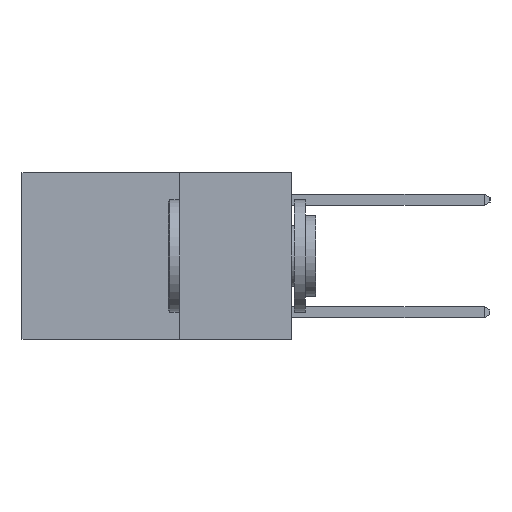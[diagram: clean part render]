
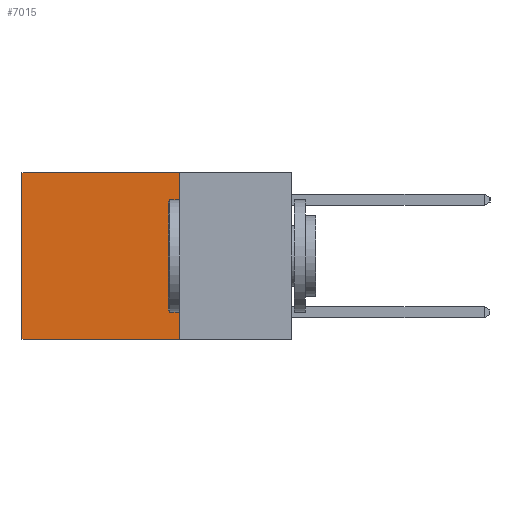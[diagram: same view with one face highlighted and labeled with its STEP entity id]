
A CAD part, left-side view. The second image highlights one B-rep face of the part: STEP entity #7015.
In plain terms, the highlighted planar face has unit normal (-1, 0, 0).
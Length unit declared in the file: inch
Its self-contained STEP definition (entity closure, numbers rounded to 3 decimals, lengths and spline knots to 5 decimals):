
#33 = ORIENTED_EDGE ( 'NONE', *, *, #1955, .F. ) ;
#361 = VERTEX_POINT ( 'NONE', #7771 ) ;
#423 = VERTEX_POINT ( 'NONE', #7670 ) ;
#875 = EDGE_LOOP ( 'NONE', ( #1395, #33, #5418, #2627 ) ) ;
#1241 = EDGE_CURVE ( 'NONE', #361, #423, #3917, .T. ) ;
#1385 = DIRECTION ( 'NONE',  ( 0., 0., -1. ) ) ;
#1395 = ORIENTED_EDGE ( 'NONE', *, *, #8363, .T. ) ;
#1513 = FACE_OUTER_BOUND ( 'NONE', #875, .T. ) ;
#1831 = CARTESIAN_POINT ( 'NONE',  ( 0.2625, 0.25, -0.37 ) ) ;
#1955 = EDGE_CURVE ( 'NONE', #423, #8313, #3493, .T. ) ;
#2224 = CARTESIAN_POINT ( 'NONE',  ( 0.2625, 0.25, 0. ) ) ;
#2562 = CARTESIAN_POINT ( 'NONE',  ( 0.2625, 0.6, -0.37 ) ) ;
#2627 = ORIENTED_EDGE ( 'NONE', *, *, #4364, .T. ) ;
#3493 = LINE ( 'NONE', #1831, #3540 ) ;
#3540 = VECTOR ( 'NONE', #7913, 39.37008 ) ;
#3891 = VECTOR ( 'NONE', #7590, 39.37008 ) ;
#3917 = LINE ( 'NONE', #5654, #3891 ) ;
#4248 = CARTESIAN_POINT ( 'NONE',  ( 0.2625, 0.25, 0. ) ) ;
#4364 = EDGE_CURVE ( 'NONE', #361, #4371, #7109, .T. ) ;
#4371 = VERTEX_POINT ( 'NONE', #6617 ) ;
#5418 = ORIENTED_EDGE ( 'NONE', *, *, #1241, .F. ) ;
#5654 = CARTESIAN_POINT ( 'NONE',  ( 0.2625, 0.25, 0. ) ) ;
#5785 = PLANE ( 'NONE',  #8905 ) ;
#6170 = LINE ( 'NONE', #8759, #6378 ) ;
#6378 = VECTOR ( 'NONE', #1385, 39.37008 ) ;
#6617 = CARTESIAN_POINT ( 'NONE',  ( 0.2625, 0.6, 0. ) ) ;
#6626 = DIRECTION ( 'NONE',  ( 0., 1., 0. ) ) ;
#6672 = DIRECTION ( 'NONE',  ( 1., 0., 0. ) ) ;
#7006 = VECTOR ( 'NONE', #6626, 39.37008 ) ;
#7015 = ADVANCED_FACE ( 'NONE', ( #1513 ), #5785, .F. ) ;
#7031 = DIRECTION ( 'NONE',  ( 0., 0., -1. ) ) ;
#7109 = LINE ( 'NONE', #4248, #7006 ) ;
#7590 = DIRECTION ( 'NONE',  ( 0., 0., -1. ) ) ;
#7670 = CARTESIAN_POINT ( 'NONE',  ( 0.2625, 0.25, -0.37 ) ) ;
#7771 = CARTESIAN_POINT ( 'NONE',  ( 0.2625, 0.25, 0. ) ) ;
#7913 = DIRECTION ( 'NONE',  ( 0., 1., 0. ) ) ;
#8313 = VERTEX_POINT ( 'NONE', #2562 ) ;
#8363 = EDGE_CURVE ( 'NONE', #4371, #8313, #6170, .T. ) ;
#8759 = CARTESIAN_POINT ( 'NONE',  ( 0.2625, 0.6, 0. ) ) ;
#8905 = AXIS2_PLACEMENT_3D ( 'NONE', #2224, #6672, #7031 ) ;
